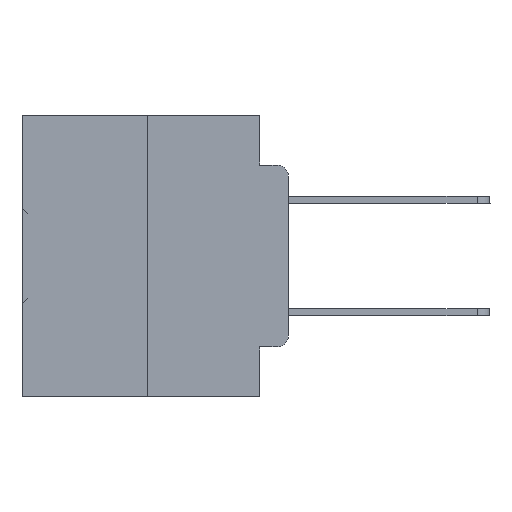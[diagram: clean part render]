
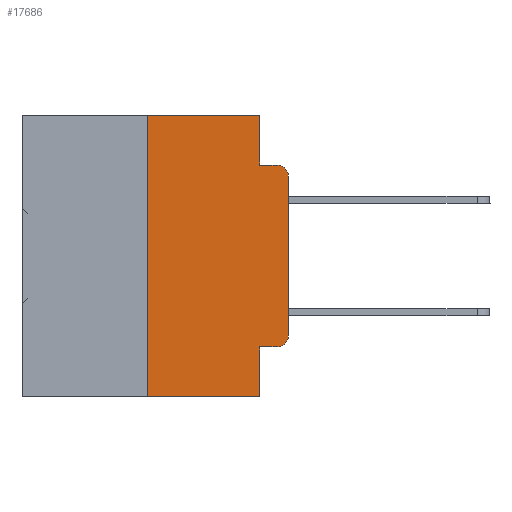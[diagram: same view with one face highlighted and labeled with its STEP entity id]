
A CAD part, left-side view. The second image highlights one B-rep face of the part: STEP entity #17686.
In plain terms, the highlighted planar face has unit normal (-1, 0, 0).
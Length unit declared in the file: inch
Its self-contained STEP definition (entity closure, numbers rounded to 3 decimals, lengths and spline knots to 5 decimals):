
#1213 = VERTEX_POINT ( 'NONE', #32016 ) ;
#1369 = CARTESIAN_POINT ( 'NONE',  ( 0., 0., 0. ) ) ;
#1414 = DIRECTION ( 'NONE',  ( 0., 0., -1. ) ) ;
#1551 = AXIS2_PLACEMENT_3D ( 'NONE', #37735, #19617, #1414 ) ;
#1618 = CARTESIAN_POINT ( 'NONE',  ( 0., 0.473, -0.5 ) ) ;
#1734 = CARTESIAN_POINT ( 'NONE',  ( 0., 0., -0.3915 ) ) ;
#1747 = DIRECTION ( 'NONE',  ( 0., -1., 0. ) ) ;
#2043 = EDGE_CURVE ( 'NONE', #8609, #27015, #22827, .T. ) ;
#4363 = VERTEX_POINT ( 'NONE', #1734 ) ;
#4501 = CARTESIAN_POINT ( 'NONE',  ( 0., 0.051, -0.4115 ) ) ;
#4866 = ORIENTED_EDGE ( 'NONE', *, *, #30404, .T. ) ;
#4929 = EDGE_CURVE ( 'NONE', #37469, #27624, #30868, .T. ) ;
#5375 = DIRECTION ( 'NONE',  ( 0., 0., 1. ) ) ;
#6817 = EDGE_CURVE ( 'NONE', #35030, #23692, #33291, .T. ) ;
#8609 = VERTEX_POINT ( 'NONE', #29164 ) ;
#8912 = ORIENTED_EDGE ( 'NONE', *, *, #19013, .T. ) ;
#11021 = CARTESIAN_POINT ( 'NONE',  ( 0., 0.473, 0. ) ) ;
#11467 = VECTOR ( 'NONE', #24524, 39.37008 ) ;
#12262 = ORIENTED_EDGE ( 'NONE', *, *, #35355, .F. ) ;
#13573 = CARTESIAN_POINT ( 'NONE',  ( 0., 0.02, -0.4115 ) ) ;
#13771 = VECTOR ( 'NONE', #1747, 39.37008 ) ;
#13810 = LINE ( 'NONE', #22990, #27088 ) ;
#13878 = EDGE_CURVE ( 'NONE', #35924, #27015, #33639, .T. ) ;
#14437 = AXIS2_PLACEMENT_3D ( 'NONE', #11021, #32612, #26291 ) ;
#14953 = CARTESIAN_POINT ( 'NONE',  ( 0., 0.051, -0.0885 ) ) ;
#15337 = DIRECTION ( 'NONE',  ( 0., 0., -1. ) ) ;
#15541 = CIRCLE ( 'NONE', #1551, 0.02 ) ;
#16188 = VERTEX_POINT ( 'NONE', #13573 ) ;
#16447 = DIRECTION ( 'NONE',  ( -1., 0., 0. ) ) ;
#16571 = DIRECTION ( 'NONE',  ( 0., -1., 0. ) ) ;
#16930 = LINE ( 'NONE', #26857, #25015 ) ;
#17686 = ADVANCED_FACE ( 'NONE', ( #28525 ), #23634, .F. ) ;
#17942 = ORIENTED_EDGE ( 'NONE', *, *, #4929, .T. ) ;
#18555 = CARTESIAN_POINT ( 'NONE',  ( 0., 0., -0.1085 ) ) ;
#18776 = ORIENTED_EDGE ( 'NONE', *, *, #6817, .F. ) ;
#19012 = DIRECTION ( 'NONE',  ( 0., 0., 1. ) ) ;
#19013 = EDGE_CURVE ( 'NONE', #16188, #4363, #15541, .T. ) ;
#19168 = VECTOR ( 'NONE', #19012, 39.37008 ) ;
#19600 = CARTESIAN_POINT ( 'NONE',  ( 0., 0.051, 0. ) ) ;
#19617 = DIRECTION ( 'NONE',  ( -1., 0., 0. ) ) ;
#20605 = CARTESIAN_POINT ( 'NONE',  ( 0., 0.25, -0.5 ) ) ;
#20970 = EDGE_LOOP ( 'NONE', ( #4866, #17942, #28813, #18776, #26187, #12262, #31702, #21461, #21517, #8912 ) ) ;
#21461 = ORIENTED_EDGE ( 'NONE', *, *, #2043, .F. ) ;
#21517 = ORIENTED_EDGE ( 'NONE', *, *, #36500, .T. ) ;
#22242 = EDGE_CURVE ( 'NONE', #23692, #27624, #27613, .T. ) ;
#22295 = CARTESIAN_POINT ( 'NONE',  ( 0., 0.051, 0. ) ) ;
#22827 = LINE ( 'NONE', #22295, #29010 ) ;
#22990 = CARTESIAN_POINT ( 'NONE',  ( 0., 0.473, 0. ) ) ;
#23634 = PLANE ( 'NONE',  #14437 ) ;
#23692 = VERTEX_POINT ( 'NONE', #14953 ) ;
#23809 = VECTOR ( 'NONE', #37170, 39.37008 ) ;
#24524 = DIRECTION ( 'NONE',  ( 0., -1., 0. ) ) ;
#24904 = LINE ( 'NONE', #4501, #26796 ) ;
#25015 = VECTOR ( 'NONE', #5375, 39.37008 ) ;
#25497 = CARTESIAN_POINT ( 'NONE',  ( 0., 0.02, -0.1085 ) ) ;
#26120 = CARTESIAN_POINT ( 'NONE',  ( 0., 0.02, -0.0885 ) ) ;
#26187 = ORIENTED_EDGE ( 'NONE', *, *, #32742, .F. ) ;
#26291 = DIRECTION ( 'NONE',  ( 0., 0., -1. ) ) ;
#26796 = VECTOR ( 'NONE', #16571, 39.37008 ) ;
#26857 = CARTESIAN_POINT ( 'NONE',  ( 0., 0.25, 0. ) ) ;
#27015 = VERTEX_POINT ( 'NONE', #32370 ) ;
#27088 = VECTOR ( 'NONE', #29098, 39.37008 ) ;
#27613 = LINE ( 'NONE', #28077, #11467 ) ;
#27624 = VERTEX_POINT ( 'NONE', #26120 ) ;
#28039 = AXIS2_PLACEMENT_3D ( 'NONE', #25497, #16447, #34347 ) ;
#28077 = CARTESIAN_POINT ( 'NONE',  ( 0., 0.051, -0.0885 ) ) ;
#28525 = FACE_OUTER_BOUND ( 'NONE', #20970, .T. ) ;
#28813 = ORIENTED_EDGE ( 'NONE', *, *, #22242, .F. ) ;
#29010 = VECTOR ( 'NONE', #15337, 39.37008 ) ;
#29098 = DIRECTION ( 'NONE',  ( 0., -1., 0. ) ) ;
#29164 = CARTESIAN_POINT ( 'NONE',  ( 0., 0.051, -0.4115 ) ) ;
#30404 = EDGE_CURVE ( 'NONE', #4363, #37469, #33864, .T. ) ;
#30868 = CIRCLE ( 'NONE', #28039, 0.02 ) ;
#30991 = CARTESIAN_POINT ( 'NONE',  ( 0., 0.051, 0. ) ) ;
#31702 = ORIENTED_EDGE ( 'NONE', *, *, #13878, .T. ) ;
#32016 = CARTESIAN_POINT ( 'NONE',  ( 0., 0.25, 0. ) ) ;
#32370 = CARTESIAN_POINT ( 'NONE',  ( 0., 0.051, -0.5 ) ) ;
#32612 = DIRECTION ( 'NONE',  ( 1., 0., 0. ) ) ;
#32742 = EDGE_CURVE ( 'NONE', #1213, #35030, #13810, .T. ) ;
#33291 = LINE ( 'NONE', #30991, #23809 ) ;
#33639 = LINE ( 'NONE', #1618, #13771 ) ;
#33864 = LINE ( 'NONE', #1369, #19168 ) ;
#34347 = DIRECTION ( 'NONE',  ( 0., 0., -1. ) ) ;
#35030 = VERTEX_POINT ( 'NONE', #19600 ) ;
#35355 = EDGE_CURVE ( 'NONE', #35924, #1213, #16930, .T. ) ;
#35924 = VERTEX_POINT ( 'NONE', #20605 ) ;
#36500 = EDGE_CURVE ( 'NONE', #8609, #16188, #24904, .T. ) ;
#37170 = DIRECTION ( 'NONE',  ( 0., 0., -1. ) ) ;
#37469 = VERTEX_POINT ( 'NONE', #18555 ) ;
#37735 = CARTESIAN_POINT ( 'NONE',  ( 0., 0.02, -0.3915 ) ) ;
